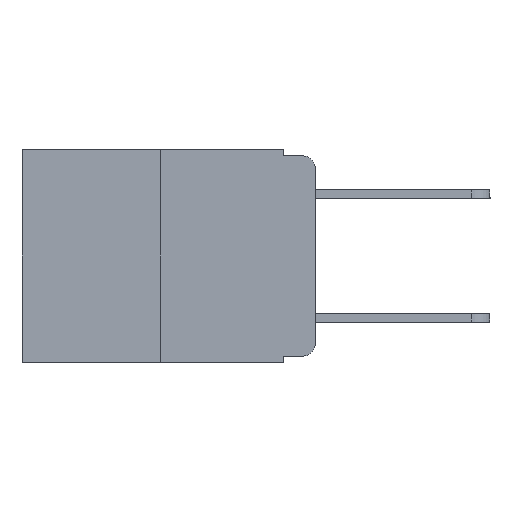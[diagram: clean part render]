
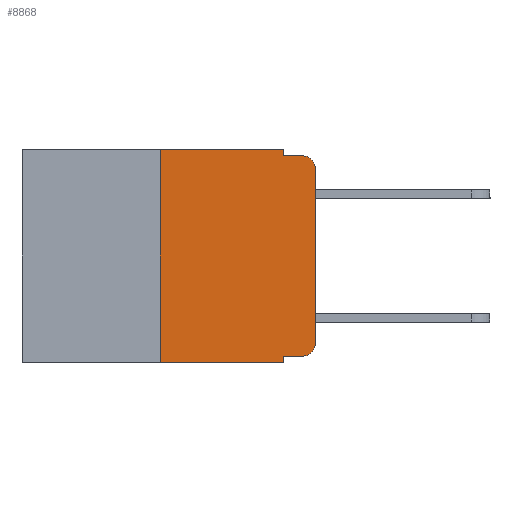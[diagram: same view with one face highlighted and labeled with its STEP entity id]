
A CAD part, left-side view. The second image highlights one B-rep face of the part: STEP entity #8868.
In plain terms, the highlighted planar face has unit normal (-1, 0, 0).
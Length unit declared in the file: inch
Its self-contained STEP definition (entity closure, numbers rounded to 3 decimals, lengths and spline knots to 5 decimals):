
#421 = AXIS2_PLACEMENT_3D ( 'NONE', #22572, #11133, #24481 ) ;
#549 = DIRECTION ( 'NONE',  ( -1., 0., 0. ) ) ;
#745 = ORIENTED_EDGE ( 'NONE', *, *, #21338, .F. ) ;
#1851 = EDGE_CURVE ( 'NONE', #7959, #11805, #9081, .T. ) ;
#2364 = EDGE_CURVE ( 'NONE', #11335, #17560, #16836, .T. ) ;
#2643 = ORIENTED_EDGE ( 'NONE', *, *, #11270, .F. ) ;
#2723 = EDGE_CURVE ( 'NONE', #7646, #17560, #19203, .T. ) ;
#3329 = VECTOR ( 'NONE', #11935, 39.37008 ) ;
#3608 = CARTESIAN_POINT ( 'NONE',  ( 0., 0.051, -0.333 ) ) ;
#3741 = LINE ( 'NONE', #24389, #13436 ) ;
#3743 = CARTESIAN_POINT ( 'NONE',  ( 0., 0.051, -0.343 ) ) ;
#3902 = ORIENTED_EDGE ( 'NONE', *, *, #23902, .F. ) ;
#4220 = ORIENTED_EDGE ( 'NONE', *, *, #8524, .F. ) ;
#4280 = VERTEX_POINT ( 'NONE', #11636 ) ;
#4760 = CARTESIAN_POINT ( 'NONE',  ( 0., 0.051, -0.333 ) ) ;
#4931 = ORIENTED_EDGE ( 'NONE', *, *, #13968, .T. ) ;
#5638 = LINE ( 'NONE', #19152, #15287 ) ;
#5701 = DIRECTION ( 'NONE',  ( 0., 0., -1. ) ) ;
#6718 = ORIENTED_EDGE ( 'NONE', *, *, #2723, .F. ) ;
#7306 = VECTOR ( 'NONE', #21690, 39.37008 ) ;
#7340 = LINE ( 'NONE', #23283, #3329 ) ;
#7636 = CARTESIAN_POINT ( 'NONE',  ( 0., 0.02, -0.01 ) ) ;
#7646 = VERTEX_POINT ( 'NONE', #3608 ) ;
#7655 = VECTOR ( 'NONE', #12533, 39.37008 ) ;
#7882 = CARTESIAN_POINT ( 'NONE',  ( 0., 0.051, 0. ) ) ;
#7906 = LINE ( 'NONE', #19764, #7306 ) ;
#7908 = DIRECTION ( 'NONE',  ( 0., -1., 0. ) ) ;
#7959 = VERTEX_POINT ( 'NONE', #18137 ) ;
#8246 = CARTESIAN_POINT ( 'NONE',  ( 0., 0., -0.313 ) ) ;
#8524 = EDGE_CURVE ( 'NONE', #4280, #11805, #7906, .T. ) ;
#8831 = VERTEX_POINT ( 'NONE', #9123 ) ;
#8868 = ADVANCED_FACE ( 'NONE', ( #16339 ), #9295, .F. ) ;
#9081 = CIRCLE ( 'NONE', #421, 0.02 ) ;
#9123 = CARTESIAN_POINT ( 'NONE',  ( 0., 0.02, -0.333 ) ) ;
#9295 = PLANE ( 'NONE',  #20274 ) ;
#9841 = CARTESIAN_POINT ( 'NONE',  ( 0., 0.473, 0. ) ) ;
#10619 = CARTESIAN_POINT ( 'NONE',  ( 0., 0.473, -0.343 ) ) ;
#11133 = DIRECTION ( 'NONE',  ( -1., 0., 0. ) ) ;
#11232 = DIRECTION ( 'NONE',  ( 0., 0., -1. ) ) ;
#11270 = EDGE_CURVE ( 'NONE', #14887, #23240, #21588, .T. ) ;
#11335 = VERTEX_POINT ( 'NONE', #21471 ) ;
#11636 = CARTESIAN_POINT ( 'NONE',  ( 0., 0.051, -0.01 ) ) ;
#11735 = VECTOR ( 'NONE', #18300, 39.37008 ) ;
#11805 = VERTEX_POINT ( 'NONE', #7636 ) ;
#11875 = CARTESIAN_POINT ( 'NONE',  ( 0., 0.051, 0. ) ) ;
#11935 = DIRECTION ( 'NONE',  ( 0., 0., 1. ) ) ;
#12313 = CARTESIAN_POINT ( 'NONE',  ( 0., 0.02, -0.313 ) ) ;
#12401 = AXIS2_PLACEMENT_3D ( 'NONE', #12313, #549, #14236 ) ;
#12533 = DIRECTION ( 'NONE',  ( 0., -1., 0. ) ) ;
#13318 = ORIENTED_EDGE ( 'NONE', *, *, #2364, .T. ) ;
#13436 = VECTOR ( 'NONE', #14879, 39.37008 ) ;
#13968 = EDGE_CURVE ( 'NONE', #7646, #8831, #22344, .T. ) ;
#14236 = DIRECTION ( 'NONE',  ( 0., 0., -1. ) ) ;
#14879 = DIRECTION ( 'NONE',  ( 0., 0., 1. ) ) ;
#14887 = VERTEX_POINT ( 'NONE', #15498 ) ;
#15287 = VECTOR ( 'NONE', #5701, 39.37008 ) ;
#15367 = CIRCLE ( 'NONE', #12401, 0.02 ) ;
#15498 = CARTESIAN_POINT ( 'NONE',  ( 0., 0.25, 0. ) ) ;
#16004 = ORIENTED_EDGE ( 'NONE', *, *, #1851, .T. ) ;
#16339 = FACE_OUTER_BOUND ( 'NONE', #20123, .T. ) ;
#16836 = LINE ( 'NONE', #10619, #11735 ) ;
#16981 = ORIENTED_EDGE ( 'NONE', *, *, #17830, .T. ) ;
#17121 = VERTEX_POINT ( 'NONE', #8246 ) ;
#17560 = VERTEX_POINT ( 'NONE', #3743 ) ;
#17579 = ORIENTED_EDGE ( 'NONE', *, *, #21826, .T. ) ;
#17830 = EDGE_CURVE ( 'NONE', #8831, #17121, #15367, .T. ) ;
#18137 = CARTESIAN_POINT ( 'NONE',  ( 0., 0., -0.03 ) ) ;
#18300 = DIRECTION ( 'NONE',  ( 0., -1., 0. ) ) ;
#19152 = CARTESIAN_POINT ( 'NONE',  ( 0., 0.051, 0. ) ) ;
#19203 = LINE ( 'NONE', #7882, #24291 ) ;
#19764 = CARTESIAN_POINT ( 'NONE',  ( 0., 0.051, -0.01 ) ) ;
#20123 = EDGE_LOOP ( 'NONE', ( #17579, #16004, #4220, #745, #2643, #3902, #13318, #6718, #4931, #16981 ) ) ;
#20274 = AXIS2_PLACEMENT_3D ( 'NONE', #20755, #22674, #11232 ) ;
#20392 = VECTOR ( 'NONE', #7908, 39.37008 ) ;
#20755 = CARTESIAN_POINT ( 'NONE',  ( 0., 0.473, 0. ) ) ;
#21275 = DIRECTION ( 'NONE',  ( 0., 0., -1. ) ) ;
#21338 = EDGE_CURVE ( 'NONE', #23240, #4280, #5638, .T. ) ;
#21471 = CARTESIAN_POINT ( 'NONE',  ( 0., 0.25, -0.343 ) ) ;
#21588 = LINE ( 'NONE', #9841, #20392 ) ;
#21690 = DIRECTION ( 'NONE',  ( 0., -1., 0. ) ) ;
#21826 = EDGE_CURVE ( 'NONE', #17121, #7959, #3741, .T. ) ;
#22344 = LINE ( 'NONE', #4760, #7655 ) ;
#22572 = CARTESIAN_POINT ( 'NONE',  ( 0., 0.02, -0.03 ) ) ;
#22674 = DIRECTION ( 'NONE',  ( 1., 0., 0. ) ) ;
#23240 = VERTEX_POINT ( 'NONE', #11875 ) ;
#23283 = CARTESIAN_POINT ( 'NONE',  ( 0., 0.25, 0. ) ) ;
#23902 = EDGE_CURVE ( 'NONE', #11335, #14887, #7340, .T. ) ;
#24291 = VECTOR ( 'NONE', #21275, 39.37008 ) ;
#24389 = CARTESIAN_POINT ( 'NONE',  ( 0., 0., 0. ) ) ;
#24481 = DIRECTION ( 'NONE',  ( 0., 0., -1. ) ) ;
